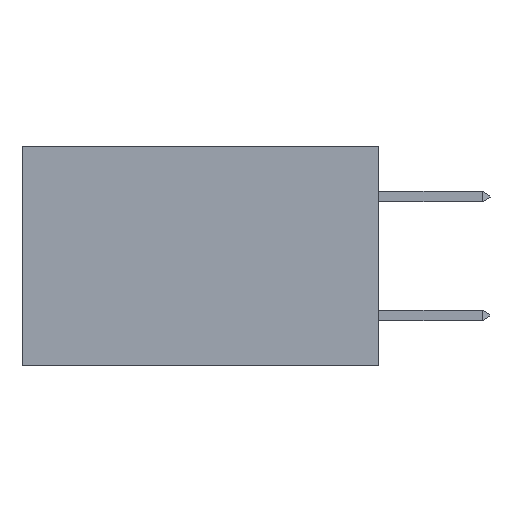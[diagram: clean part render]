
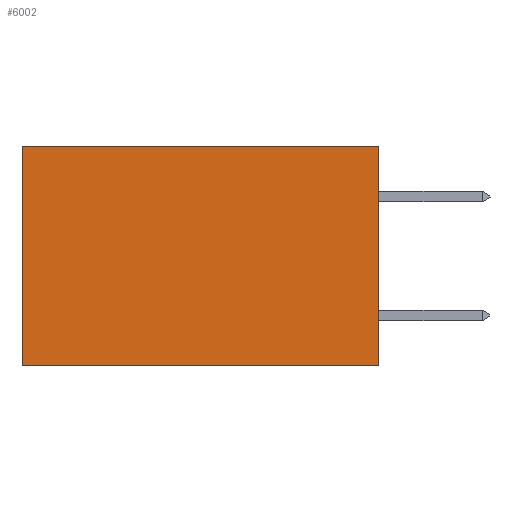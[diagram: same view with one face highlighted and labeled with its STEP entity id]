
A CAD part, left-side view. The second image highlights one B-rep face of the part: STEP entity #6002.
In plain terms, the highlighted planar face has unit normal (-1, 0, 0).
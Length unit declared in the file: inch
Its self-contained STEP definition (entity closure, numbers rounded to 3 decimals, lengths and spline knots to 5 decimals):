
#1747 = VERTEX_POINT ( 'NONE', #16625 ) ;
#1795 = CARTESIAN_POINT ( 'NONE',  ( 0.298, 0.6, 0. ) ) ;
#2204 = LINE ( 'NONE', #22368, #14209 ) ;
#2444 = LINE ( 'NONE', #18655, #21844 ) ;
#3370 = EDGE_CURVE ( 'NONE', #14690, #1747, #2204, .T. ) ;
#4392 = DIRECTION ( 'NONE',  ( 0., 0., -1. ) ) ;
#6002 = ADVANCED_FACE ( 'NONE', ( #9296 ), #12168, .F. ) ;
#6477 = EDGE_CURVE ( 'NONE', #10532, #28276, #2444, .T. ) ;
#6608 = CARTESIAN_POINT ( 'NONE',  ( 0.298, 0.6, 0. ) ) ;
#7053 = LINE ( 'NONE', #1795, #25507 ) ;
#8448 = CARTESIAN_POINT ( 'NONE',  ( 0.298, 0., 0. ) ) ;
#9296 = FACE_OUTER_BOUND ( 'NONE', #14987, .T. ) ;
#10532 = VERTEX_POINT ( 'NONE', #8448 ) ;
#12168 = PLANE ( 'NONE',  #30867 ) ;
#12856 = ORIENTED_EDGE ( 'NONE', *, *, #3370, .F. ) ;
#14081 = DIRECTION ( 'NONE',  ( 0., 0., -1. ) ) ;
#14209 = VECTOR ( 'NONE', #15144, 39.37008 ) ;
#14304 = ORIENTED_EDGE ( 'NONE', *, *, #22449, .T. ) ;
#14690 = VERTEX_POINT ( 'NONE', #23988 ) ;
#14987 = EDGE_LOOP ( 'NONE', ( #14304, #12856, #27608, #20252 ) ) ;
#15064 = VECTOR ( 'NONE', #20807, 39.37008 ) ;
#15144 = DIRECTION ( 'NONE',  ( 0., 1., 0. ) ) ;
#16625 = CARTESIAN_POINT ( 'NONE',  ( 0.298, 0.6, -0.37 ) ) ;
#17121 = DIRECTION ( 'NONE',  ( 1., 0., 0. ) ) ;
#18655 = CARTESIAN_POINT ( 'NONE',  ( 0.298, 0., 0. ) ) ;
#20252 = ORIENTED_EDGE ( 'NONE', *, *, #6477, .T. ) ;
#20807 = DIRECTION ( 'NONE',  ( 0., 0., -1. ) ) ;
#21844 = VECTOR ( 'NONE', #31428, 39.37008 ) ;
#22368 = CARTESIAN_POINT ( 'NONE',  ( 0.298, 0., -0.37 ) ) ;
#22449 = EDGE_CURVE ( 'NONE', #28276, #1747, #7053, .T. ) ;
#23988 = CARTESIAN_POINT ( 'NONE',  ( 0.298, 0., -0.37 ) ) ;
#25507 = VECTOR ( 'NONE', #4392, 39.37008 ) ;
#27608 = ORIENTED_EDGE ( 'NONE', *, *, #29340, .F. ) ;
#28229 = LINE ( 'NONE', #30582, #15064 ) ;
#28276 = VERTEX_POINT ( 'NONE', #6608 ) ;
#29340 = EDGE_CURVE ( 'NONE', #10532, #14690, #28229, .T. ) ;
#30582 = CARTESIAN_POINT ( 'NONE',  ( 0.298, 0., 0. ) ) ;
#30867 = AXIS2_PLACEMENT_3D ( 'NONE', #31289, #17121, #14081 ) ;
#31289 = CARTESIAN_POINT ( 'NONE',  ( 0.298, 0., 0. ) ) ;
#31428 = DIRECTION ( 'NONE',  ( 0., 1., 0. ) ) ;
